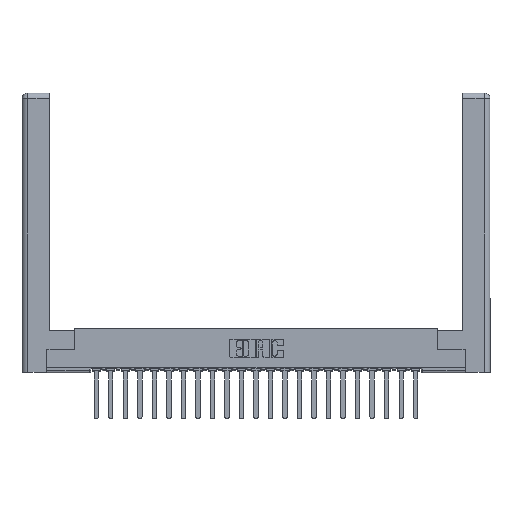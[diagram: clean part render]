
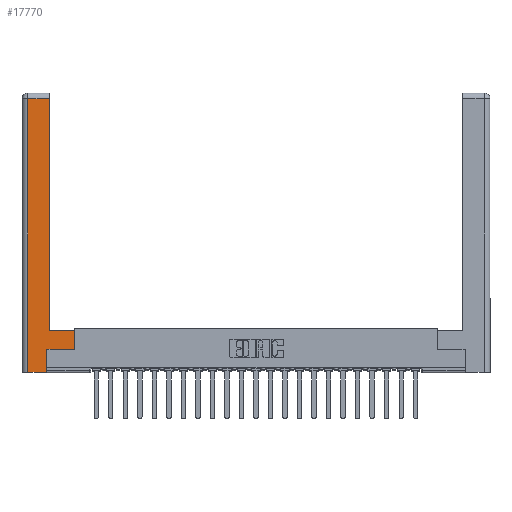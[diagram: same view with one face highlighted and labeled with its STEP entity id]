
A CAD part, top view. The second image highlights one B-rep face of the part: STEP entity #17770.
In plain terms, the highlighted planar face has unit normal (0, 0, 1).
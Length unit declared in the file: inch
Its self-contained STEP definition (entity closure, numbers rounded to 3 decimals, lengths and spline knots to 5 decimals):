
#760 = ORIENTED_EDGE ( 'NONE', *, *, #17484, .T. ) ;
#2004 = EDGE_CURVE ( 'NONE', #15017, #17516, #23086, .T. ) ;
#2935 = LINE ( 'NONE', #21997, #14070 ) ;
#3853 = DIRECTION ( 'NONE',  ( 0., -1., 0. ) ) ;
#5402 = LINE ( 'NONE', #9140, #17862 ) ;
#6023 = DIRECTION ( 'NONE',  ( 0., 0., -1. ) ) ;
#6861 = VERTEX_POINT ( 'NONE', #9793 ) ;
#7230 = VECTOR ( 'NONE', #11263, 39.37008 ) ;
#7277 = VERTEX_POINT ( 'NONE', #7581 ) ;
#7581 = CARTESIAN_POINT ( 'NONE',  ( 0.295, 2.94, 0. ) ) ;
#7711 = VERTEX_POINT ( 'NONE', #11532 ) ;
#7834 = ORIENTED_EDGE ( 'NONE', *, *, #8855, .T. ) ;
#8034 = CARTESIAN_POINT ( 'NONE',  ( 0.565, 0.45, 0. ) ) ;
#8650 = EDGE_CURVE ( 'NONE', #6861, #12001, #2935, .T. ) ;
#8855 = EDGE_CURVE ( 'NONE', #7711, #15017, #12853, .T. ) ;
#9140 = CARTESIAN_POINT ( 'NONE',  ( 0.565, 0.245, 0. ) ) ;
#9344 = ORIENTED_EDGE ( 'NONE', *, *, #15140, .T. ) ;
#9506 = CARTESIAN_POINT ( 'NONE',  ( 0., 0., 0. ) ) ;
#9780 = EDGE_CURVE ( 'NONE', #24660, #7711, #19045, .T. ) ;
#9793 = CARTESIAN_POINT ( 'NONE',  ( 0.565, 0.245, 0. ) ) ;
#10043 = AXIS2_PLACEMENT_3D ( 'NONE', #9506, #6023, #25195 ) ;
#10846 = VECTOR ( 'NONE', #13064, 39.37008 ) ;
#11092 = VECTOR ( 'NONE', #3853, 39.37008 ) ;
#11138 = LINE ( 'NONE', #24640, #7230 ) ;
#11263 = DIRECTION ( 'NONE',  ( 0., 1., 0. ) ) ;
#11532 = CARTESIAN_POINT ( 'NONE',  ( 0.0615, 0., 0. ) ) ;
#12001 = VERTEX_POINT ( 'NONE', #8034 ) ;
#12061 = EDGE_LOOP ( 'NONE', ( #18311, #9344, #13173, #7834, #16702, #22283, #25080, #760 ) ) ;
#12390 = LINE ( 'NONE', #18321, #21483 ) ;
#12620 = CARTESIAN_POINT ( 'NONE',  ( 0.295, 0.45, 0. ) ) ;
#12853 = LINE ( 'NONE', #22765, #17129 ) ;
#13064 = DIRECTION ( 'NONE',  ( 0., 1., 0. ) ) ;
#13173 = ORIENTED_EDGE ( 'NONE', *, *, #9780, .T. ) ;
#13494 = PLANE ( 'NONE',  #10043 ) ;
#13497 = CARTESIAN_POINT ( 'NONE',  ( 0.0615, 0., 0. ) ) ;
#13916 = CARTESIAN_POINT ( 'NONE',  ( 0.0615, 2.94, 0. ) ) ;
#14070 = VECTOR ( 'NONE', #14143, 39.37008 ) ;
#14143 = DIRECTION ( 'NONE',  ( 0., 1., 0. ) ) ;
#14671 = DIRECTION ( 'NONE',  ( -1., 0., 0. ) ) ;
#15017 = VERTEX_POINT ( 'NONE', #17558 ) ;
#15140 = EDGE_CURVE ( 'NONE', #7277, #24660, #12390, .T. ) ;
#15375 = CARTESIAN_POINT ( 'NONE',  ( 0.265, 0.245, 0. ) ) ;
#16382 = DIRECTION ( 'NONE',  ( -1., 0., 0. ) ) ;
#16702 = ORIENTED_EDGE ( 'NONE', *, *, #2004, .T. ) ;
#17025 = VECTOR ( 'NONE', #14671, 39.37008 ) ;
#17129 = VECTOR ( 'NONE', #24813, 39.37008 ) ;
#17237 = DIRECTION ( 'NONE',  ( 1., 0., 0. ) ) ;
#17484 = EDGE_CURVE ( 'NONE', #12001, #18749, #22135, .T. ) ;
#17516 = VERTEX_POINT ( 'NONE', #18408 ) ;
#17555 = CARTESIAN_POINT ( 'NONE',  ( 0.295, 0.45, 0. ) ) ;
#17558 = CARTESIAN_POINT ( 'NONE',  ( 0.265, 0., 0. ) ) ;
#17659 = EDGE_CURVE ( 'NONE', #17516, #6861, #5402, .T. ) ;
#17770 = ADVANCED_FACE ( 'NONE', ( #19279 ), #13494, .F. ) ;
#17862 = VECTOR ( 'NONE', #17237, 39.37008 ) ;
#18311 = ORIENTED_EDGE ( 'NONE', *, *, #19798, .T. ) ;
#18321 = CARTESIAN_POINT ( 'NONE',  ( 0.0615, 2.94, 0. ) ) ;
#18408 = CARTESIAN_POINT ( 'NONE',  ( 0.265, 0.245, 0. ) ) ;
#18749 = VERTEX_POINT ( 'NONE', #17555 ) ;
#19045 = LINE ( 'NONE', #13497, #11092 ) ;
#19279 = FACE_OUTER_BOUND ( 'NONE', #12061, .T. ) ;
#19798 = EDGE_CURVE ( 'NONE', #18749, #7277, #11138, .T. ) ;
#21483 = VECTOR ( 'NONE', #16382, 39.37008 ) ;
#21997 = CARTESIAN_POINT ( 'NONE',  ( 0.565, 0.45, 0. ) ) ;
#22135 = LINE ( 'NONE', #12620, #17025 ) ;
#22283 = ORIENTED_EDGE ( 'NONE', *, *, #17659, .T. ) ;
#22765 = CARTESIAN_POINT ( 'NONE',  ( 0.265, 0., 0. ) ) ;
#23086 = LINE ( 'NONE', #15375, #10846 ) ;
#24640 = CARTESIAN_POINT ( 'NONE',  ( 0.295, 3., 0. ) ) ;
#24660 = VERTEX_POINT ( 'NONE', #13916 ) ;
#24813 = DIRECTION ( 'NONE',  ( 1., 0., 0. ) ) ;
#25080 = ORIENTED_EDGE ( 'NONE', *, *, #8650, .T. ) ;
#25195 = DIRECTION ( 'NONE',  ( -1., 0., 0. ) ) ;
